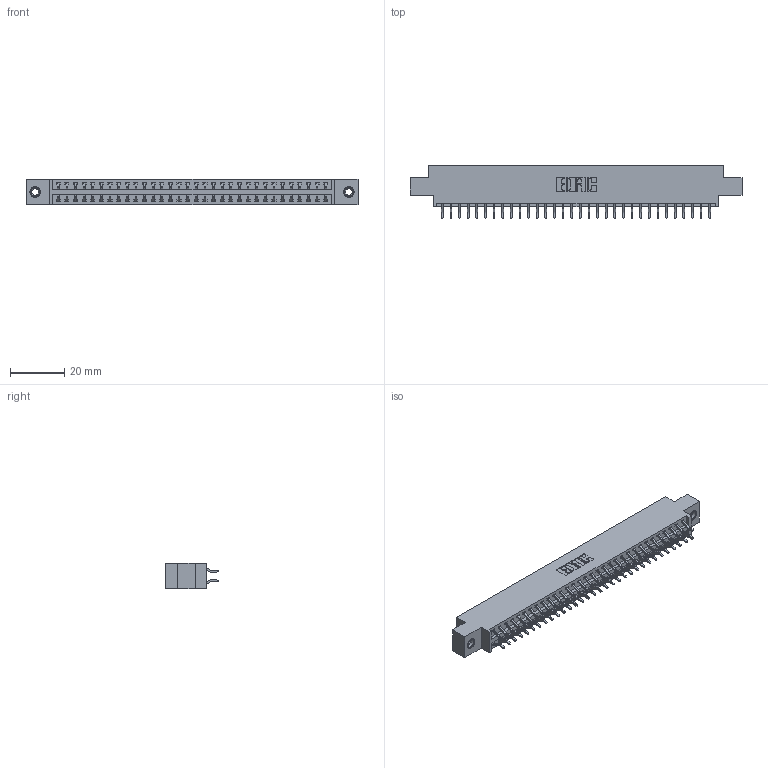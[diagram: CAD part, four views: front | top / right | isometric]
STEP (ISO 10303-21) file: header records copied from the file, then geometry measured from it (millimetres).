
FILE_DESCRIPTION (( 'STEP AP203' ), '1' );
FILE_NAME ('346-064-556-807.STEP', '2018-08-28T09:34:51', ( '' ), ( '' ), 'SwSTEP 2.0', 'SolidWorks 2016', '' );
FILE_SCHEMA (( 'CONFIG_CONTROL_DESIGN' ));
Length unit declared in the file: inch
Products named in the file (4): 345-292-001_556 Tail; 345-250-001_345-250-005-103; 346-064-556-807; 346 Part_0.170 Offset - 0.156 Dia-TI
Assembly tree (67 placements, depth 2):
  346-064-556-807
    346 Part_0.170 Offset - 0.156 Dia-TI
    345-292-001_556 Tail  x64
    345-250-001_345-250-005-103  x2
Bounding box: 122.17 x 19.57 x 9.4 mm (x, y, z)
Volume: 11665.2 mm3; surface area: 16031.3 mm2
Topology: 67 solids, 67 shells, 3898 faces, 11549 edges, 7606 vertices
Faces by surface type: plane 2608, cylinder 1274, cone 12, torus 4
Entity records: 23768 total; most frequent: CARTESIAN_POINT 3931, ORIENTED_EDGE 3846, DIRECTION 3529, EDGE_CURVE 1923, VECTOR 1635, LINE 1635, VERTEX_POINT 1276, AXIS2_PLACEMENT_3D 947
